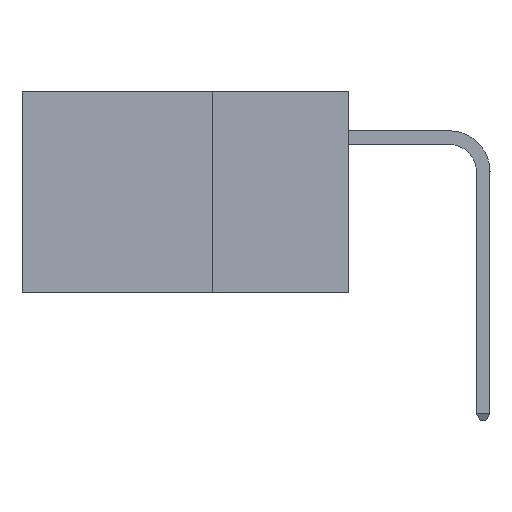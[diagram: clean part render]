
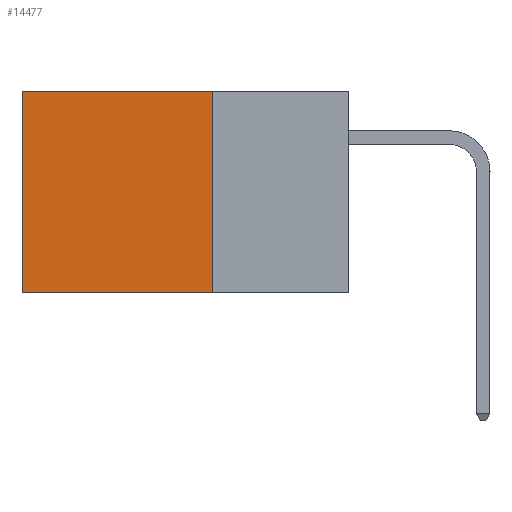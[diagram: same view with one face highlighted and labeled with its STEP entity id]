
A CAD part, left-side view. The second image highlights one B-rep face of the part: STEP entity #14477.
In plain terms, the highlighted planar face has unit normal (-1, 0, 0).
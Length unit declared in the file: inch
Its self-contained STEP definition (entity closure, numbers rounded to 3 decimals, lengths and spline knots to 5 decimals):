
#78 = DIRECTION ( 'NONE',  ( 0., 1., 0. ) ) ;
#934 = CARTESIAN_POINT ( 'NONE',  ( 0.2875, 0.6, -0.37 ) ) ;
#3063 = DIRECTION ( 'NONE',  ( 0., 0., -1. ) ) ;
#3300 = DIRECTION ( 'NONE',  ( 1., 0., 0. ) ) ;
#3558 = EDGE_CURVE ( 'NONE', #13147, #24348, #44594, .T. ) ;
#3749 = VECTOR ( 'NONE', #32598, 39.37008 ) ;
#4058 = AXIS2_PLACEMENT_3D ( 'NONE', #32965, #3300, #14390 ) ;
#4476 = ORIENTED_EDGE ( 'NONE', *, *, #3558, .T. ) ;
#4624 = VECTOR ( 'NONE', #3063, 39.37008 ) ;
#6641 = EDGE_CURVE ( 'NONE', #42260, #21899, #19227, .T. ) ;
#10626 = DIRECTION ( 'NONE',  ( 0., 1., 0. ) ) ;
#12204 = VECTOR ( 'NONE', #10626, 39.37008 ) ;
#12890 = CARTESIAN_POINT ( 'NONE',  ( 0.2875, 0.6, 0. ) ) ;
#13147 = VERTEX_POINT ( 'NONE', #22971 ) ;
#14338 = ORIENTED_EDGE ( 'NONE', *, *, #6641, .F. ) ;
#14390 = DIRECTION ( 'NONE',  ( 0., 0., -1. ) ) ;
#14477 = ADVANCED_FACE ( 'NONE', ( #31087 ), #18457, .F. ) ;
#15016 = LINE ( 'NONE', #22412, #27272 ) ;
#18457 = PLANE ( 'NONE',  #4058 ) ;
#19227 = LINE ( 'NONE', #36787, #4624 ) ;
#19432 = ORIENTED_EDGE ( 'NONE', *, *, #35987, .F. ) ;
#21899 = VERTEX_POINT ( 'NONE', #24678 ) ;
#22412 = CARTESIAN_POINT ( 'NONE',  ( 0.2875, 0.25, -0.37 ) ) ;
#22971 = CARTESIAN_POINT ( 'NONE',  ( 0.2875, 0.6, 0. ) ) ;
#24348 = VERTEX_POINT ( 'NONE', #934 ) ;
#24678 = CARTESIAN_POINT ( 'NONE',  ( 0.2875, 0.25, -0.37 ) ) ;
#27272 = VECTOR ( 'NONE', #78, 39.37008 ) ;
#27361 = LINE ( 'NONE', #29052, #12204 ) ;
#29052 = CARTESIAN_POINT ( 'NONE',  ( 0.2875, 0.25, 0. ) ) ;
#31087 = FACE_OUTER_BOUND ( 'NONE', #32590, .T. ) ;
#32590 = EDGE_LOOP ( 'NONE', ( #4476, #19432, #14338, #43874 ) ) ;
#32598 = DIRECTION ( 'NONE',  ( 0., 0., -1. ) ) ;
#32965 = CARTESIAN_POINT ( 'NONE',  ( 0.2875, 0.25, 0. ) ) ;
#35199 = EDGE_CURVE ( 'NONE', #42260, #13147, #27361, .T. ) ;
#35987 = EDGE_CURVE ( 'NONE', #21899, #24348, #15016, .T. ) ;
#36787 = CARTESIAN_POINT ( 'NONE',  ( 0.2875, 0.25, 0. ) ) ;
#39596 = CARTESIAN_POINT ( 'NONE',  ( 0.2875, 0.25, 0. ) ) ;
#42260 = VERTEX_POINT ( 'NONE', #39596 ) ;
#43874 = ORIENTED_EDGE ( 'NONE', *, *, #35199, .T. ) ;
#44594 = LINE ( 'NONE', #12890, #3749 ) ;
